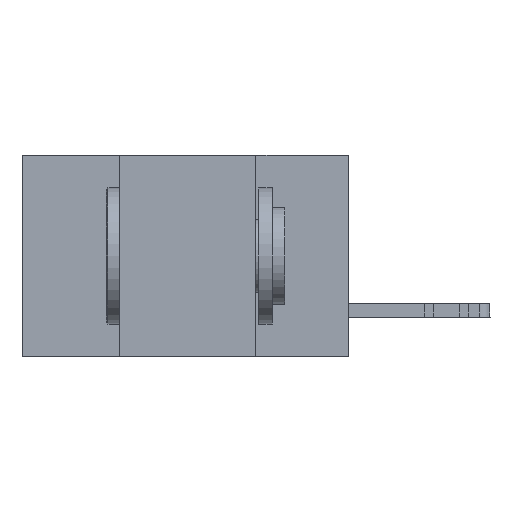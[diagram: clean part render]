
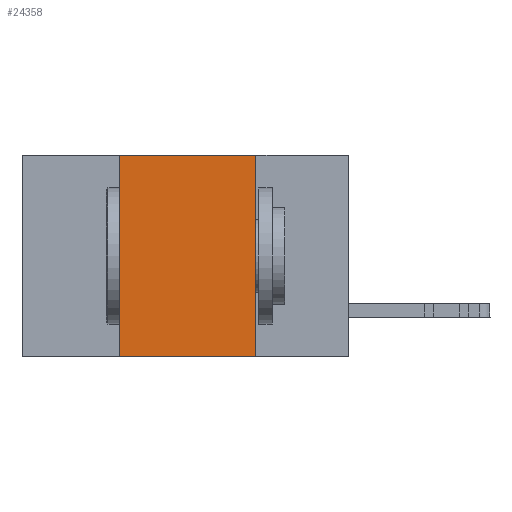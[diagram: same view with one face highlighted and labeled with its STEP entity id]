
A CAD part, left-side view. The second image highlights one B-rep face of the part: STEP entity #24358.
In plain terms, the highlighted planar face has unit normal (-1, 0, 0).
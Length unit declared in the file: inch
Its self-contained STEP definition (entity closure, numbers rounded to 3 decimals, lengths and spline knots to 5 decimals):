
#400 = DIRECTION ( 'NONE',  ( 0., 0., -1. ) ) ;
#1324 = DIRECTION ( 'NONE',  ( 0., -1., 0. ) ) ;
#1512 = CARTESIAN_POINT ( 'NONE',  ( 0., 0.6, 0. ) ) ;
#2737 = EDGE_CURVE ( 'NONE', #20437, #7945, #7648, .T. ) ;
#4328 = ORIENTED_EDGE ( 'NONE', *, *, #22533, .F. ) ;
#7648 = LINE ( 'NONE', #21303, #18984 ) ;
#7665 = CARTESIAN_POINT ( 'NONE',  ( 0., 0.6, -0.37 ) ) ;
#7945 = VERTEX_POINT ( 'NONE', #25507 ) ;
#8203 = VECTOR ( 'NONE', #24845, 39.37008 ) ;
#8226 = CARTESIAN_POINT ( 'NONE',  ( 0., 0.42, -0.37 ) ) ;
#8533 = VECTOR ( 'NONE', #1324, 39.37008 ) ;
#8670 = VECTOR ( 'NONE', #21912, 39.37008 ) ;
#10910 = CARTESIAN_POINT ( 'NONE',  ( 0., 0.17, 0. ) ) ;
#12550 = FACE_OUTER_BOUND ( 'NONE', #25159, .T. ) ;
#14322 = LINE ( 'NONE', #10910, #8670 ) ;
#14961 = ORIENTED_EDGE ( 'NONE', *, *, #24598, .F. ) ;
#15361 = DIRECTION ( 'NONE',  ( 1., 0., 0. ) ) ;
#16114 = EDGE_CURVE ( 'NONE', #20437, #26129, #26261, .T. ) ;
#17401 = CARTESIAN_POINT ( 'NONE',  ( 0., 0.6, 0. ) ) ;
#17594 = PLANE ( 'NONE',  #18812 ) ;
#17800 = VERTEX_POINT ( 'NONE', #21405 ) ;
#18812 = AXIS2_PLACEMENT_3D ( 'NONE', #17401, #15361, #400 ) ;
#18922 = CARTESIAN_POINT ( 'NONE',  ( 0., 0.17, -0.37 ) ) ;
#18984 = VECTOR ( 'NONE', #20724, 39.37008 ) ;
#19342 = ORIENTED_EDGE ( 'NONE', *, *, #16114, .T. ) ;
#20437 = VERTEX_POINT ( 'NONE', #8226 ) ;
#20515 = LINE ( 'NONE', #1512, #8533 ) ;
#20724 = DIRECTION ( 'NONE',  ( 0., 0., 1. ) ) ;
#20928 = ORIENTED_EDGE ( 'NONE', *, *, #2737, .F. ) ;
#21303 = CARTESIAN_POINT ( 'NONE',  ( 0., 0.42, 0. ) ) ;
#21405 = CARTESIAN_POINT ( 'NONE',  ( 0., 0.17, 0. ) ) ;
#21912 = DIRECTION ( 'NONE',  ( 0., 0., -1. ) ) ;
#22533 = EDGE_CURVE ( 'NONE', #17800, #26129, #14322, .T. ) ;
#24358 = ADVANCED_FACE ( 'NONE', ( #12550 ), #17594, .F. ) ;
#24598 = EDGE_CURVE ( 'NONE', #7945, #17800, #20515, .T. ) ;
#24845 = DIRECTION ( 'NONE',  ( 0., -1., 0. ) ) ;
#25159 = EDGE_LOOP ( 'NONE', ( #4328, #14961, #20928, #19342 ) ) ;
#25507 = CARTESIAN_POINT ( 'NONE',  ( 0., 0.42, 0. ) ) ;
#26129 = VERTEX_POINT ( 'NONE', #18922 ) ;
#26261 = LINE ( 'NONE', #7665, #8203 ) ;
